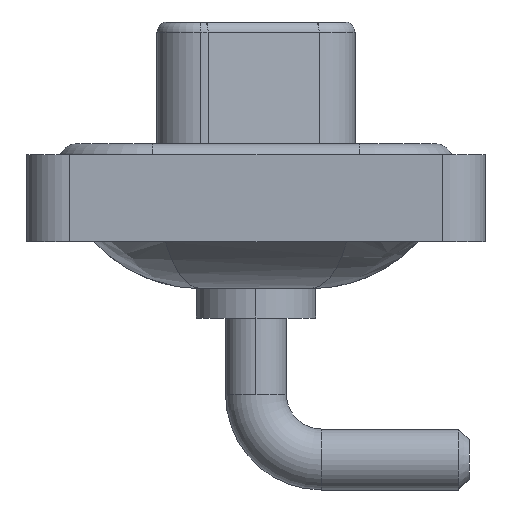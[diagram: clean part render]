
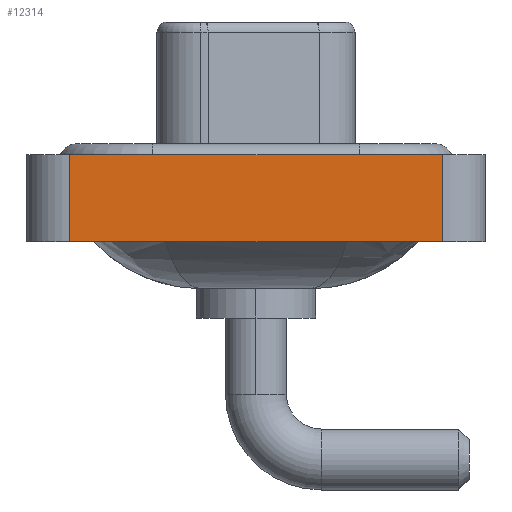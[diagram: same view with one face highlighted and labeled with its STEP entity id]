
A CAD part, left-side view. The second image highlights one B-rep face of the part: STEP entity #12314.
In plain terms, the highlighted planar face has unit normal (-1, 0, 0).
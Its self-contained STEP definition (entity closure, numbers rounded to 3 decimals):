
#336 = CARTESIAN_POINT ( 'NONE',  ( -7.35, -8.55, -3.6 ) ) ;
#408 = EDGE_CURVE ( 'NONE', #14694, #3561, #6553, .T. ) ;
#1812 = ORIENTED_EDGE ( 'NONE', *, *, #7538, .T. ) ;
#2273 = DIRECTION ( 'NONE',  ( 0., -1., 0. ) ) ;
#3561 = VERTEX_POINT ( 'NONE', #12277 ) ;
#4106 = PLANE ( 'NONE',  #8434 ) ;
#5172 = CARTESIAN_POINT ( 'NONE',  ( -7.35, 8.55, -3.6 ) ) ;
#5202 = DIRECTION ( 'NONE',  ( 0., 0., 1. ) ) ;
#6404 = LINE ( 'NONE', #13061, #7732 ) ;
#6553 = LINE ( 'NONE', #5172, #13735 ) ;
#6717 = ORIENTED_EDGE ( 'NONE', *, *, #408, .F. ) ;
#7538 = EDGE_CURVE ( 'NONE', #8402, #12372, #14779, .T. ) ;
#7732 = VECTOR ( 'NONE', #10165, 1000. ) ;
#8005 = ORIENTED_EDGE ( 'NONE', *, *, #8669, .F. ) ;
#8402 = VERTEX_POINT ( 'NONE', #13801 ) ;
#8434 = AXIS2_PLACEMENT_3D ( 'NONE', #336, #15676, #10056 ) ;
#8669 = EDGE_CURVE ( 'NONE', #3561, #12372, #6404, .T. ) ;
#8916 = VECTOR ( 'NONE', #2273, 1000. ) ;
#9272 = CARTESIAN_POINT ( 'NONE',  ( -7.35, -8.55, -3.6 ) ) ;
#9513 = CARTESIAN_POINT ( 'NONE',  ( -7.35, -8.55, -3.6 ) ) ;
#9742 = VECTOR ( 'NONE', #5202, 1000. ) ;
#10056 = DIRECTION ( 'NONE',  ( 0., 0., 1. ) ) ;
#10165 = DIRECTION ( 'NONE',  ( 0., -1., 0. ) ) ;
#11425 = CARTESIAN_POINT ( 'NONE',  ( -7.35, -8.55, 0.4 ) ) ;
#12206 = DIRECTION ( 'NONE',  ( 0., 0., 1. ) ) ;
#12277 = CARTESIAN_POINT ( 'NONE',  ( -7.35, 8.55, 0.4 ) ) ;
#12314 = ADVANCED_FACE ( 'NONE', ( #16600 ), #4106, .T. ) ;
#12372 = VERTEX_POINT ( 'NONE', #11425 ) ;
#13061 = CARTESIAN_POINT ( 'NONE',  ( -7.35, -8.55, 0.4 ) ) ;
#13735 = VECTOR ( 'NONE', #12206, 1000. ) ;
#13801 = CARTESIAN_POINT ( 'NONE',  ( -7.35, -8.55, -3.6 ) ) ;
#14694 = VERTEX_POINT ( 'NONE', #15852 ) ;
#14779 = LINE ( 'NONE', #9513, #9742 ) ;
#14889 = LINE ( 'NONE', #9272, #8916 ) ;
#14934 = ORIENTED_EDGE ( 'NONE', *, *, #16068, .T. ) ;
#15214 = EDGE_LOOP ( 'NONE', ( #1812, #8005, #6717, #14934 ) ) ;
#15676 = DIRECTION ( 'NONE',  ( -1., 0., 0. ) ) ;
#15852 = CARTESIAN_POINT ( 'NONE',  ( -7.35, 8.55, -3.6 ) ) ;
#16068 = EDGE_CURVE ( 'NONE', #14694, #8402, #14889, .T. ) ;
#16600 = FACE_OUTER_BOUND ( 'NONE', #15214, .T. ) ;
